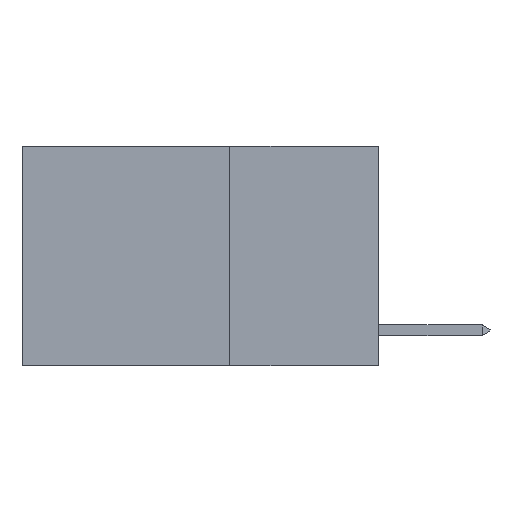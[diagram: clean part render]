
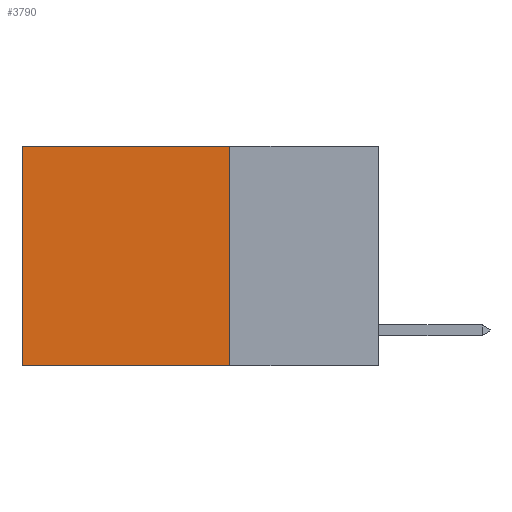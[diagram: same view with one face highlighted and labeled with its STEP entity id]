
A CAD part, left-side view. The second image highlights one B-rep face of the part: STEP entity #3790.
In plain terms, the highlighted planar face has unit normal (-1, 0, 0).
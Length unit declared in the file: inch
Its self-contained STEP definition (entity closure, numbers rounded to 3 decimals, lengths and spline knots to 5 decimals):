
#216 = EDGE_CURVE ( 'NONE', #3542, #10923, #4141, .T. ) ;
#517 = DIRECTION ( 'NONE',  ( 0., 0., -1. ) ) ;
#559 = CARTESIAN_POINT ( 'NONE',  ( 0.2625, 0.25, 0. ) ) ;
#851 = AXIS2_PLACEMENT_3D ( 'NONE', #12089, #5816, #13164 ) ;
#1285 = CARTESIAN_POINT ( 'NONE',  ( 0.2625, 0.6, 0. ) ) ;
#1630 = EDGE_LOOP ( 'NONE', ( #8479, #7122, #13104, #13387 ) ) ;
#1808 = LINE ( 'NONE', #559, #4269 ) ;
#2385 = LINE ( 'NONE', #2720, #7646 ) ;
#2720 = CARTESIAN_POINT ( 'NONE',  ( 0.2625, 0.25, 0. ) ) ;
#3152 = EDGE_CURVE ( 'NONE', #11098, #3542, #2385, .T. ) ;
#3542 = VERTEX_POINT ( 'NONE', #1285 ) ;
#3764 = DIRECTION ( 'NONE',  ( 0., 1., 0. ) ) ;
#3790 = ADVANCED_FACE ( 'NONE', ( #13364 ), #4753, .F. ) ;
#3966 = LINE ( 'NONE', #6535, #8591 ) ;
#4141 = LINE ( 'NONE', #12319, #11839 ) ;
#4269 = VECTOR ( 'NONE', #517, 39.37008 ) ;
#4753 = PLANE ( 'NONE',  #851 ) ;
#5170 = EDGE_CURVE ( 'NONE', #6167, #10923, #3966, .T. ) ;
#5816 = DIRECTION ( 'NONE',  ( 1., 0., 0. ) ) ;
#5963 = EDGE_CURVE ( 'NONE', #11098, #6167, #1808, .T. ) ;
#6167 = VERTEX_POINT ( 'NONE', #11382 ) ;
#6535 = CARTESIAN_POINT ( 'NONE',  ( 0.2625, 0.25, -0.37 ) ) ;
#7122 = ORIENTED_EDGE ( 'NONE', *, *, #5170, .F. ) ;
#7646 = VECTOR ( 'NONE', #3764, 39.37008 ) ;
#7668 = CARTESIAN_POINT ( 'NONE',  ( 0.2625, 0.6, -0.37 ) ) ;
#8479 = ORIENTED_EDGE ( 'NONE', *, *, #216, .T. ) ;
#8591 = VECTOR ( 'NONE', #8728, 39.37008 ) ;
#8728 = DIRECTION ( 'NONE',  ( 0., 1., 0. ) ) ;
#10923 = VERTEX_POINT ( 'NONE', #7668 ) ;
#11098 = VERTEX_POINT ( 'NONE', #12082 ) ;
#11382 = CARTESIAN_POINT ( 'NONE',  ( 0.2625, 0.25, -0.37 ) ) ;
#11839 = VECTOR ( 'NONE', #12157, 39.37008 ) ;
#12082 = CARTESIAN_POINT ( 'NONE',  ( 0.2625, 0.25, 0. ) ) ;
#12089 = CARTESIAN_POINT ( 'NONE',  ( 0.2625, 0.25, 0. ) ) ;
#12157 = DIRECTION ( 'NONE',  ( 0., 0., -1. ) ) ;
#12319 = CARTESIAN_POINT ( 'NONE',  ( 0.2625, 0.6, 0. ) ) ;
#13104 = ORIENTED_EDGE ( 'NONE', *, *, #5963, .F. ) ;
#13164 = DIRECTION ( 'NONE',  ( 0., 0., -1. ) ) ;
#13364 = FACE_OUTER_BOUND ( 'NONE', #1630, .T. ) ;
#13387 = ORIENTED_EDGE ( 'NONE', *, *, #3152, .T. ) ;
